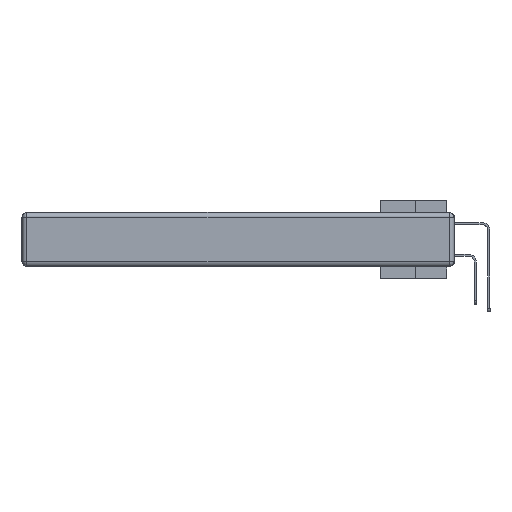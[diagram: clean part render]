
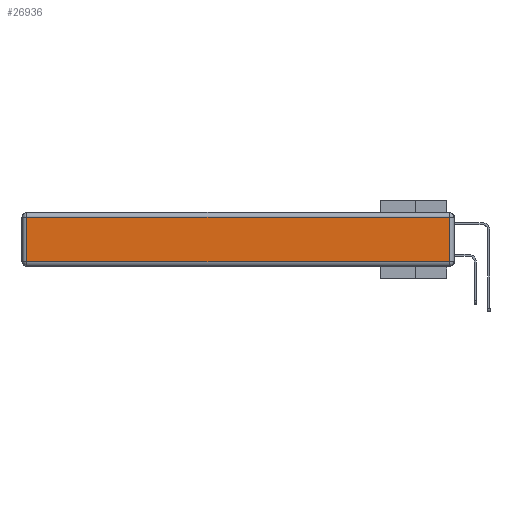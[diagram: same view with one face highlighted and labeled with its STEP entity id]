
A CAD part, left-side view. The second image highlights one B-rep face of the part: STEP entity #26936.
In plain terms, the highlighted planar face has unit normal (-1, 0, 0).
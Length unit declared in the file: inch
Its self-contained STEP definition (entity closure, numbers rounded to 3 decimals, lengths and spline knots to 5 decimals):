
#854 = DIRECTION ( 'NONE',  ( -1., 0., 0. ) ) ;
#1545 = LINE ( 'NONE', #22356, #19772 ) ;
#5560 = ORIENTED_EDGE ( 'NONE', *, *, #26546, .T. ) ;
#7741 = VECTOR ( 'NONE', #23677, 39.37008 ) ;
#8193 = CARTESIAN_POINT ( 'NONE',  ( 0., 0.03, -0.03 ) ) ;
#8240 = AXIS2_PLACEMENT_3D ( 'NONE', #23594, #854, #26657 ) ;
#8912 = LINE ( 'NONE', #35496, #23483 ) ;
#9004 = EDGE_CURVE ( 'NONE', #37402, #32746, #14732, .T. ) ;
#11066 = EDGE_LOOP ( 'NONE', ( #35056, #31168, #5560, #26600 ) ) ;
#11844 = CARTESIAN_POINT ( 'NONE',  ( 0., 2.72, -0.343 ) ) ;
#12005 = LINE ( 'NONE', #26548, #7741 ) ;
#12484 = PLANE ( 'NONE',  #8240 ) ;
#13556 = CARTESIAN_POINT ( 'NONE',  ( 0., 0.03, -0.313 ) ) ;
#14732 = LINE ( 'NONE', #11844, #21331 ) ;
#14741 = VERTEX_POINT ( 'NONE', #13556 ) ;
#16305 = EDGE_CURVE ( 'NONE', #32746, #14741, #12005, .T. ) ;
#18342 = VERTEX_POINT ( 'NONE', #8193 ) ;
#19486 = DIRECTION ( 'NONE',  ( 0., 0., 1. ) ) ;
#19772 = VECTOR ( 'NONE', #19486, 39.37008 ) ;
#21324 = DIRECTION ( 'NONE',  ( 0., 1., 0. ) ) ;
#21331 = VECTOR ( 'NONE', #35195, 39.37008 ) ;
#22356 = CARTESIAN_POINT ( 'NONE',  ( 0., 0.03, -0.343 ) ) ;
#23483 = VECTOR ( 'NONE', #21324, 39.37008 ) ;
#23594 = CARTESIAN_POINT ( 'NONE',  ( 0., 0., -0.343 ) ) ;
#23677 = DIRECTION ( 'NONE',  ( 0., -1., 0. ) ) ;
#25789 = EDGE_CURVE ( 'NONE', #14741, #18342, #1545, .T. ) ;
#26546 = EDGE_CURVE ( 'NONE', #18342, #37402, #8912, .T. ) ;
#26548 = CARTESIAN_POINT ( 'NONE',  ( 0., 0., -0.313 ) ) ;
#26600 = ORIENTED_EDGE ( 'NONE', *, *, #9004, .T. ) ;
#26657 = DIRECTION ( 'NONE',  ( 0., 0., 1. ) ) ;
#26936 = ADVANCED_FACE ( 'NONE', ( #27036 ), #12484, .T. ) ;
#27036 = FACE_OUTER_BOUND ( 'NONE', #11066, .T. ) ;
#31168 = ORIENTED_EDGE ( 'NONE', *, *, #25789, .T. ) ;
#32746 = VERTEX_POINT ( 'NONE', #34566 ) ;
#34566 = CARTESIAN_POINT ( 'NONE',  ( 0., 2.72, -0.313 ) ) ;
#34958 = CARTESIAN_POINT ( 'NONE',  ( 0., 2.72, -0.03 ) ) ;
#35056 = ORIENTED_EDGE ( 'NONE', *, *, #16305, .T. ) ;
#35195 = DIRECTION ( 'NONE',  ( 0., 0., -1. ) ) ;
#35496 = CARTESIAN_POINT ( 'NONE',  ( 0., 2.75, -0.03 ) ) ;
#37402 = VERTEX_POINT ( 'NONE', #34958 ) ;
